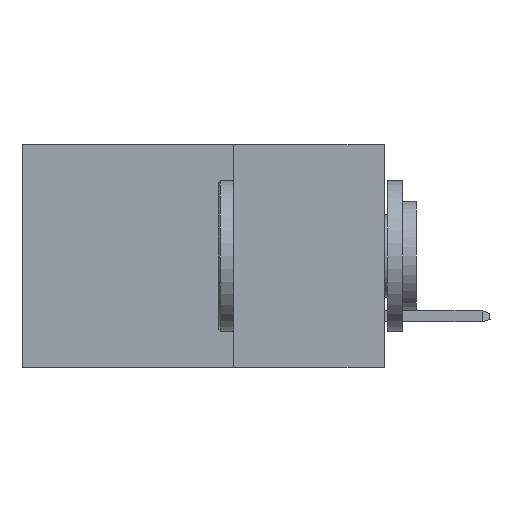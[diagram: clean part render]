
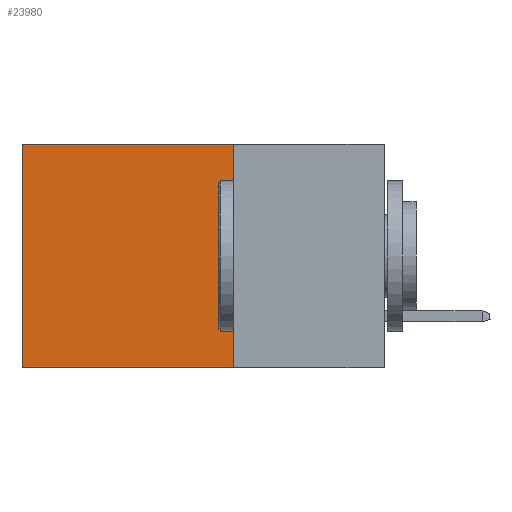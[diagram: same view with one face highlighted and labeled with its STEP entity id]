
A CAD part, left-side view. The second image highlights one B-rep face of the part: STEP entity #23980.
In plain terms, the highlighted planar face has unit normal (-1, 0, 0).
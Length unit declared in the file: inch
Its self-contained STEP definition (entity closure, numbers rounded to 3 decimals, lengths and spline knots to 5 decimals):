
#1544 = VERTEX_POINT ( 'NONE', #9347 ) ;
#1652 = CARTESIAN_POINT ( 'NONE',  ( 0.298, 0.25, 0. ) ) ;
#1762 = DIRECTION ( 'NONE',  ( 0., 1., 0. ) ) ;
#2097 = LINE ( 'NONE', #16902, #12319 ) ;
#2382 = CARTESIAN_POINT ( 'NONE',  ( 0.298, 0.25, 0. ) ) ;
#2457 = DIRECTION ( 'NONE',  ( 0., 0., -1. ) ) ;
#2736 = EDGE_CURVE ( 'NONE', #7526, #21913, #9956, .T. ) ;
#4303 = DIRECTION ( 'NONE',  ( 0., 1., 0. ) ) ;
#7526 = VERTEX_POINT ( 'NONE', #13369 ) ;
#9134 = CARTESIAN_POINT ( 'NONE',  ( 0.298, 0.6, -0.37 ) ) ;
#9165 = EDGE_CURVE ( 'NONE', #1544, #7526, #22712, .T. ) ;
#9347 = CARTESIAN_POINT ( 'NONE',  ( 0.298, 0.25, 0. ) ) ;
#9956 = LINE ( 'NONE', #32196, #17388 ) ;
#10942 = ORIENTED_EDGE ( 'NONE', *, *, #9165, .T. ) ;
#12129 = VERTEX_POINT ( 'NONE', #19863 ) ;
#12319 = VECTOR ( 'NONE', #4303, 39.37008 ) ;
#12830 = VECTOR ( 'NONE', #1762, 39.37008 ) ;
#13369 = CARTESIAN_POINT ( 'NONE',  ( 0.298, 0.6, 0. ) ) ;
#14421 = LINE ( 'NONE', #2382, #26679 ) ;
#14787 = DIRECTION ( 'NONE',  ( 0., 0., -1. ) ) ;
#16902 = CARTESIAN_POINT ( 'NONE',  ( 0.298, 0.25, -0.37 ) ) ;
#17388 = VECTOR ( 'NONE', #32401, 39.37008 ) ;
#19863 = CARTESIAN_POINT ( 'NONE',  ( 0.298, 0.25, -0.37 ) ) ;
#20056 = DIRECTION ( 'NONE',  ( 1., 0., 0. ) ) ;
#21913 = VERTEX_POINT ( 'NONE', #9134 ) ;
#22196 = FACE_OUTER_BOUND ( 'NONE', #23967, .T. ) ;
#22374 = EDGE_CURVE ( 'NONE', #1544, #12129, #14421, .T. ) ;
#22712 = LINE ( 'NONE', #1652, #12830 ) ;
#23366 = ORIENTED_EDGE ( 'NONE', *, *, #22374, .F. ) ;
#23372 = AXIS2_PLACEMENT_3D ( 'NONE', #27859, #20056, #2457 ) ;
#23967 = EDGE_LOOP ( 'NONE', ( #28598, #26367, #23366, #10942 ) ) ;
#23980 = ADVANCED_FACE ( 'NONE', ( #22196 ), #25233, .F. ) ;
#24387 = EDGE_CURVE ( 'NONE', #12129, #21913, #2097, .T. ) ;
#25233 = PLANE ( 'NONE',  #23372 ) ;
#26367 = ORIENTED_EDGE ( 'NONE', *, *, #24387, .F. ) ;
#26679 = VECTOR ( 'NONE', #14787, 39.37008 ) ;
#27859 = CARTESIAN_POINT ( 'NONE',  ( 0.298, 0.25, 0. ) ) ;
#28598 = ORIENTED_EDGE ( 'NONE', *, *, #2736, .T. ) ;
#32196 = CARTESIAN_POINT ( 'NONE',  ( 0.298, 0.6, 0. ) ) ;
#32401 = DIRECTION ( 'NONE',  ( 0., 0., -1. ) ) ;
